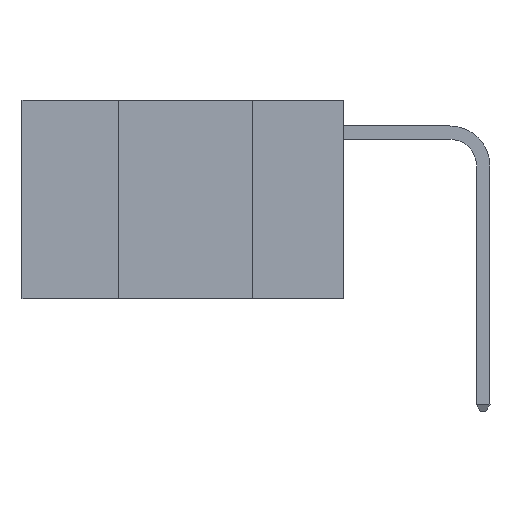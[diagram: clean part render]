
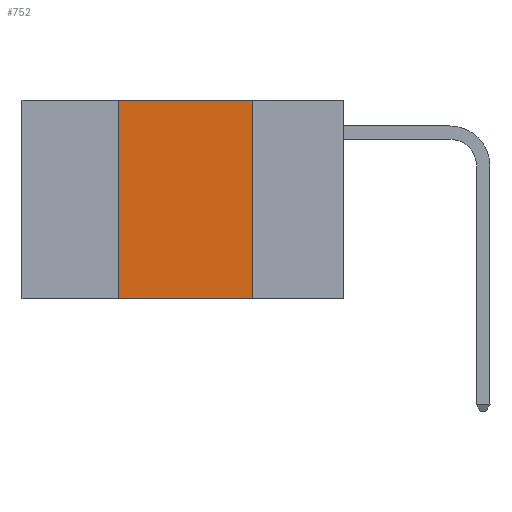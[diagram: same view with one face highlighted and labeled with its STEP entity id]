
A CAD part, left-side view. The second image highlights one B-rep face of the part: STEP entity #752.
In plain terms, the highlighted planar face has unit normal (-1, 0, 0).
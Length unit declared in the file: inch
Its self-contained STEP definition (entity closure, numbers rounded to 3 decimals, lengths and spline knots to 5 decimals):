
#33 = DIRECTION ( 'NONE',  ( 0., 0., -1. ) ) ;
#623 = DIRECTION ( 'NONE',  ( 0., -1., 0. ) ) ;
#714 = LINE ( 'NONE', #1348, #3199 ) ;
#752 = ADVANCED_FACE ( 'NONE', ( #5913 ), #7471, .F. ) ;
#896 = ORIENTED_EDGE ( 'NONE', *, *, #5367, .F. ) ;
#1182 = LINE ( 'NONE', #2540, #5908 ) ;
#1348 = CARTESIAN_POINT ( 'NONE',  ( 0., 0.42, 0. ) ) ;
#1803 = VERTEX_POINT ( 'NONE', #9391 ) ;
#1831 = AXIS2_PLACEMENT_3D ( 'NONE', #9523, #2053, #33 ) ;
#2053 = DIRECTION ( 'NONE',  ( 1., 0., 0. ) ) ;
#2112 = VECTOR ( 'NONE', #6727, 39.37008 ) ;
#2365 = CARTESIAN_POINT ( 'NONE',  ( 0., 0.42, -0.37 ) ) ;
#2540 = CARTESIAN_POINT ( 'NONE',  ( 0., 0.6, 0. ) ) ;
#2602 = VECTOR ( 'NONE', #623, 39.37008 ) ;
#3174 = ORIENTED_EDGE ( 'NONE', *, *, #4587, .F. ) ;
#3199 = VECTOR ( 'NONE', #7905, 39.37008 ) ;
#3421 = ORIENTED_EDGE ( 'NONE', *, *, #4433, .T. ) ;
#3478 = DIRECTION ( 'NONE',  ( 0., -1., 0. ) ) ;
#3569 = ORIENTED_EDGE ( 'NONE', *, *, #7829, .F. ) ;
#3862 = EDGE_LOOP ( 'NONE', ( #3174, #3569, #896, #3421 ) ) ;
#4332 = CARTESIAN_POINT ( 'NONE',  ( 0., 0.6, -0.37 ) ) ;
#4378 = VERTEX_POINT ( 'NONE', #2365 ) ;
#4433 = EDGE_CURVE ( 'NONE', #4378, #1803, #5072, .T. ) ;
#4587 = EDGE_CURVE ( 'NONE', #8356, #1803, #11526, .T. ) ;
#4754 = CARTESIAN_POINT ( 'NONE',  ( 0., 0.42, 0. ) ) ;
#5072 = LINE ( 'NONE', #4332, #2602 ) ;
#5186 = CARTESIAN_POINT ( 'NONE',  ( 0., 0.17, 0. ) ) ;
#5367 = EDGE_CURVE ( 'NONE', #4378, #10933, #714, .T. ) ;
#5847 = CARTESIAN_POINT ( 'NONE',  ( 0., 0.17, 0. ) ) ;
#5908 = VECTOR ( 'NONE', #3478, 39.37008 ) ;
#5913 = FACE_OUTER_BOUND ( 'NONE', #3862, .T. ) ;
#6727 = DIRECTION ( 'NONE',  ( 0., 0., -1. ) ) ;
#7471 = PLANE ( 'NONE',  #1831 ) ;
#7829 = EDGE_CURVE ( 'NONE', #10933, #8356, #1182, .T. ) ;
#7905 = DIRECTION ( 'NONE',  ( 0., 0., 1. ) ) ;
#8356 = VERTEX_POINT ( 'NONE', #5186 ) ;
#9391 = CARTESIAN_POINT ( 'NONE',  ( 0., 0.17, -0.37 ) ) ;
#9523 = CARTESIAN_POINT ( 'NONE',  ( 0., 0.6, 0. ) ) ;
#10933 = VERTEX_POINT ( 'NONE', #4754 ) ;
#11526 = LINE ( 'NONE', #5847, #2112 ) ;
